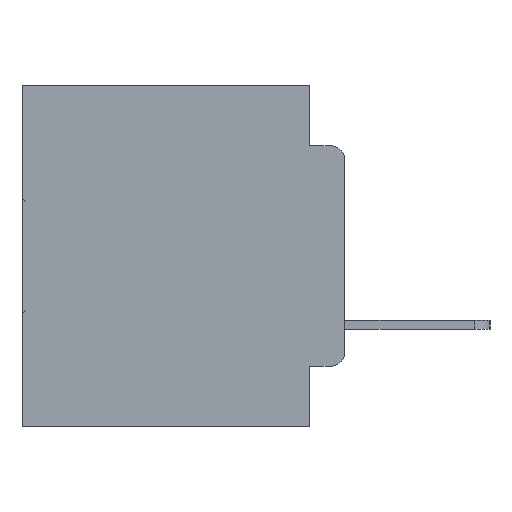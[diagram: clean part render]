
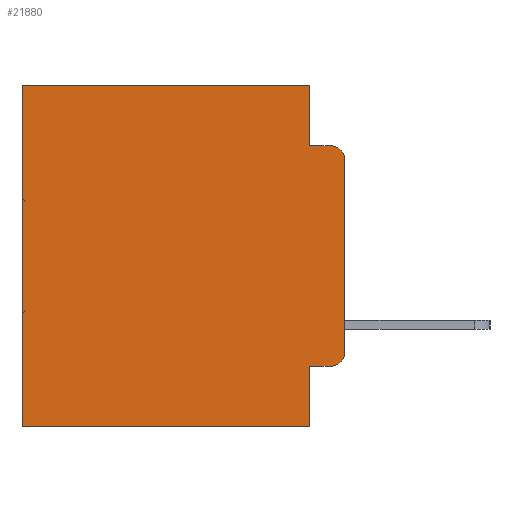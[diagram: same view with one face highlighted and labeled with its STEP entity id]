
A CAD part, left-side view. The second image highlights one B-rep face of the part: STEP entity #21880.
In plain terms, the highlighted planar face has unit normal (-1, 0, 0).
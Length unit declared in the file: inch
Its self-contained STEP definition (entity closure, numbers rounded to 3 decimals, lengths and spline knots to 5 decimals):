
#43 = PLANE ( 'NONE',  #29022 ) ;
#190 = DIRECTION ( 'NONE',  ( 1., 0., 0. ) ) ;
#1429 = DIRECTION ( 'NONE',  ( 0., 0., -1. ) ) ;
#2493 = EDGE_CURVE ( 'NONE', #26759, #9613, #4711, .T. ) ;
#2593 = ORIENTED_EDGE ( 'NONE', *, *, #14220, .T. ) ;
#3079 = LINE ( 'NONE', #6120, #17431 ) ;
#3205 = VECTOR ( 'NONE', #16036, 39.37008 ) ;
#3459 = VERTEX_POINT ( 'NONE', #19856 ) ;
#3753 = VECTOR ( 'NONE', #29525, 39.37008 ) ;
#3827 = VERTEX_POINT ( 'NONE', #12037 ) ;
#4109 = FACE_OUTER_BOUND ( 'NONE', #8143, .T. ) ;
#4466 = EDGE_CURVE ( 'NONE', #26177, #26759, #30614, .T. ) ;
#4616 = VECTOR ( 'NONE', #8280, 39.37008 ) ;
#4711 = LINE ( 'NONE', #26974, #3753 ) ;
#4788 = VERTEX_POINT ( 'NONE', #29092 ) ;
#5986 = AXIS2_PLACEMENT_3D ( 'NONE', #32927, #18512, #1429 ) ;
#6120 = CARTESIAN_POINT ( 'NONE',  ( 0.298, 0., -0.5 ) ) ;
#6829 = VECTOR ( 'NONE', #21818, 39.37008 ) ;
#6970 = ORIENTED_EDGE ( 'NONE', *, *, #2493, .F. ) ;
#7706 = DIRECTION ( 'NONE',  ( 0., 1., 0. ) ) ;
#7755 = ORIENTED_EDGE ( 'NONE', *, *, #12350, .F. ) ;
#8143 = EDGE_LOOP ( 'NONE', ( #24960, #12391, #6970, #31756, #23586, #28209, #18998, #7755, #2593, #15289 ) ) ;
#8280 = DIRECTION ( 'NONE',  ( 0., 0., -1. ) ) ;
#9613 = VERTEX_POINT ( 'NONE', #13817 ) ;
#9929 = VERTEX_POINT ( 'NONE', #31578 ) ;
#10410 = EDGE_CURVE ( 'NONE', #30986, #28839, #31241, .T. ) ;
#12037 = CARTESIAN_POINT ( 'NONE',  ( 0.298, 0.051, -0.4115 ) ) ;
#12044 = CARTESIAN_POINT ( 'NONE',  ( 0.298, 0.473, -0.5 ) ) ;
#12350 = EDGE_CURVE ( 'NONE', #3827, #4788, #15297, .T. ) ;
#12391 = ORIENTED_EDGE ( 'NONE', *, *, #32996, .T. ) ;
#12412 = VECTOR ( 'NONE', #7706, 39.37008 ) ;
#13817 = CARTESIAN_POINT ( 'NONE',  ( 0.298, 0.02, -0.0885 ) ) ;
#14220 = EDGE_CURVE ( 'NONE', #3827, #3459, #22442, .T. ) ;
#14562 = DIRECTION ( 'NONE',  ( 0., 1., 0. ) ) ;
#14675 = CARTESIAN_POINT ( 'NONE',  ( 0.298, 0.02, -0.3915 ) ) ;
#15289 = ORIENTED_EDGE ( 'NONE', *, *, #16022, .T. ) ;
#15297 = LINE ( 'NONE', #31493, #6829 ) ;
#15460 = CARTESIAN_POINT ( 'NONE',  ( 0.298, 0., -0.3915 ) ) ;
#16022 = EDGE_CURVE ( 'NONE', #3459, #18499, #19544, .T. ) ;
#16036 = DIRECTION ( 'NONE',  ( 0., 0., -1. ) ) ;
#16317 = CARTESIAN_POINT ( 'NONE',  ( 0.298, 0.051, -0.0885 ) ) ;
#17183 = CARTESIAN_POINT ( 'NONE',  ( 0.298, 0.051, 0. ) ) ;
#17374 = DIRECTION ( 'NONE',  ( 0., 0., -1. ) ) ;
#17431 = VECTOR ( 'NONE', #14562, 39.37008 ) ;
#18499 = VERTEX_POINT ( 'NONE', #15460 ) ;
#18512 = DIRECTION ( 'NONE',  ( -1., 0., 0. ) ) ;
#18760 = CARTESIAN_POINT ( 'NONE',  ( 0.298, 0.473, 0. ) ) ;
#18998 = ORIENTED_EDGE ( 'NONE', *, *, #27946, .F. ) ;
#19428 = DIRECTION ( 'NONE',  ( 0., 0., -1. ) ) ;
#19521 = LINE ( 'NONE', #26210, #12412 ) ;
#19544 = CIRCLE ( 'NONE', #20183, 0.02 ) ;
#19856 = CARTESIAN_POINT ( 'NONE',  ( 0.298, 0.02, -0.4115 ) ) ;
#19920 = DIRECTION ( 'NONE',  ( 0., 0., -1. ) ) ;
#20183 = AXIS2_PLACEMENT_3D ( 'NONE', #14675, #31979, #17374 ) ;
#20616 = CIRCLE ( 'NONE', #5986, 0.02 ) ;
#21202 = CARTESIAN_POINT ( 'NONE',  ( 0.298, 0.051, -0.4115 ) ) ;
#21610 = EDGE_CURVE ( 'NONE', #26177, #30986, #19521, .T. ) ;
#21783 = CARTESIAN_POINT ( 'NONE',  ( 0.298, 0., 0. ) ) ;
#21818 = DIRECTION ( 'NONE',  ( 0., 0., -1. ) ) ;
#21880 = ADVANCED_FACE ( 'NONE', ( #4109 ), #43, .F. ) ;
#22442 = LINE ( 'NONE', #21202, #28106 ) ;
#23382 = VECTOR ( 'NONE', #19428, 39.37008 ) ;
#23586 = ORIENTED_EDGE ( 'NONE', *, *, #21610, .T. ) ;
#23713 = DIRECTION ( 'NONE',  ( 0., -1., 0. ) ) ;
#23973 = CARTESIAN_POINT ( 'NONE',  ( 0.298, 0.473, 0. ) ) ;
#24960 = ORIENTED_EDGE ( 'NONE', *, *, #25162, .F. ) ;
#25162 = EDGE_CURVE ( 'NONE', #9929, #18499, #26860, .T. ) ;
#26177 = VERTEX_POINT ( 'NONE', #17183 ) ;
#26210 = CARTESIAN_POINT ( 'NONE',  ( 0.298, 0., 0. ) ) ;
#26759 = VERTEX_POINT ( 'NONE', #16317 ) ;
#26860 = LINE ( 'NONE', #21783, #4616 ) ;
#26974 = CARTESIAN_POINT ( 'NONE',  ( 0.298, 0.051, -0.0885 ) ) ;
#27946 = EDGE_CURVE ( 'NONE', #4788, #28839, #3079, .T. ) ;
#28106 = VECTOR ( 'NONE', #23713, 39.37008 ) ;
#28209 = ORIENTED_EDGE ( 'NONE', *, *, #10410, .T. ) ;
#28839 = VERTEX_POINT ( 'NONE', #12044 ) ;
#29022 = AXIS2_PLACEMENT_3D ( 'NONE', #31970, #190, #19920 ) ;
#29092 = CARTESIAN_POINT ( 'NONE',  ( 0.298, 0.051, -0.5 ) ) ;
#29525 = DIRECTION ( 'NONE',  ( 0., -1., 0. ) ) ;
#30614 = LINE ( 'NONE', #33735, #3205 ) ;
#30986 = VERTEX_POINT ( 'NONE', #23973 ) ;
#31241 = LINE ( 'NONE', #18760, #23382 ) ;
#31493 = CARTESIAN_POINT ( 'NONE',  ( 0.298, 0.051, 0. ) ) ;
#31578 = CARTESIAN_POINT ( 'NONE',  ( 0.298, 0., -0.1085 ) ) ;
#31756 = ORIENTED_EDGE ( 'NONE', *, *, #4466, .F. ) ;
#31970 = CARTESIAN_POINT ( 'NONE',  ( 0.298, 0., 0. ) ) ;
#31979 = DIRECTION ( 'NONE',  ( -1., 0., 0. ) ) ;
#32927 = CARTESIAN_POINT ( 'NONE',  ( 0.298, 0.02, -0.1085 ) ) ;
#32996 = EDGE_CURVE ( 'NONE', #9929, #9613, #20616, .T. ) ;
#33735 = CARTESIAN_POINT ( 'NONE',  ( 0.298, 0.051, 0. ) ) ;
